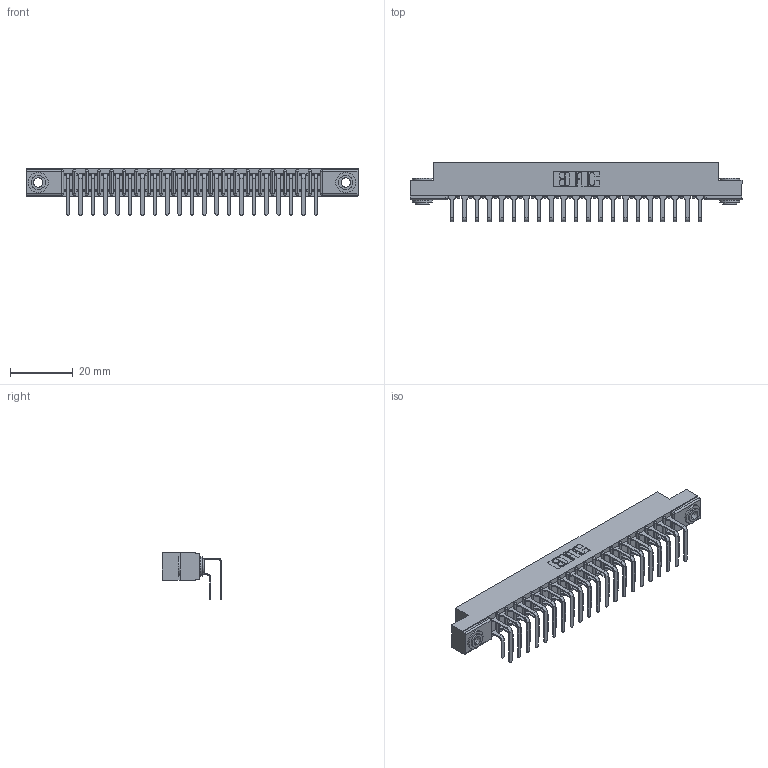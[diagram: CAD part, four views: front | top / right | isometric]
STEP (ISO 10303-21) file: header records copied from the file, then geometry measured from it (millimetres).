
FILE_DESCRIPTION (( 'STEP AP203' ), '1' );
FILE_NAME ('357-042-458-203.STEP', '2020-10-03T22:55:57', ( '' ), ( '' ), 'SwSTEP 2.0', 'SolidWorks 2020', '' );
FILE_SCHEMA (( 'CONFIG_CONTROL_DESIGN' ));
Length unit declared in the file: inch
Products named in the file (5): 345-250-002_345-250-002-102; 357-042-458-203; 307-290-001_558 - 2 (Single); 307 Part_.156 Dia Mounting Holes; 307-290-001_558 559 - 1 (Single)
Assembly tree (45 placements, depth 2):
  357-042-458-203
    307 Part_.156 Dia Mounting Holes
    307-290-001_558 559 - 1 (Single)  x21
    307-290-001_558 - 2 (Single)  x21
    345-250-002_345-250-002-102  x2
Bounding box: 106.22 x 18.96 x 14.81 mm (x, y, z)
Volume: 7135.7 mm3; surface area: 13846.7 mm2
Topology: 45 solids, 45 shells, 2292 faces, 6399 edges, 4146 vertices
Faces by surface type: plane 1480, cylinder 760, sphere 44, cone 8
Entity records: 23776 total; most frequent: CARTESIAN_POINT 3880, ORIENTED_EDGE 3834, DIRECTION 3823, EDGE_CURVE 1917, LINE 1453, VECTOR 1453, VERTEX_POINT 1242, AXIS2_PLACEMENT_3D 1185
